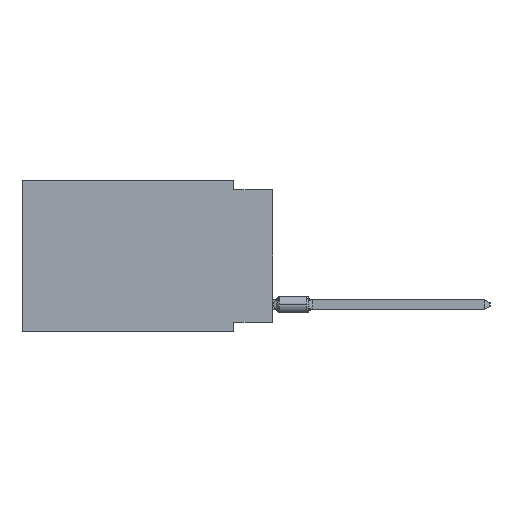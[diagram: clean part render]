
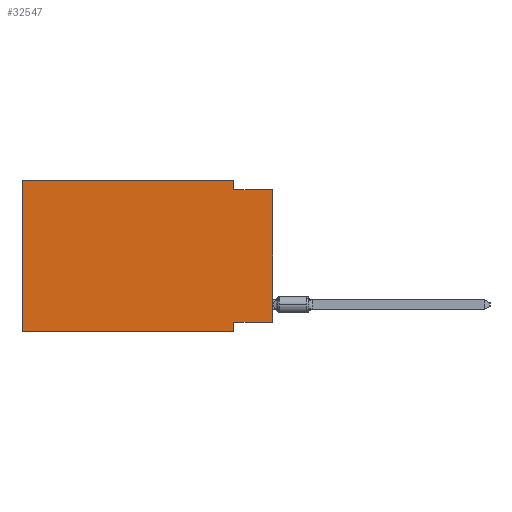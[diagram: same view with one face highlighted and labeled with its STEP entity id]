
A CAD part, left-side view. The second image highlights one B-rep face of the part: STEP entity #32547.
In plain terms, the highlighted planar face has unit normal (-1, 0, 0).
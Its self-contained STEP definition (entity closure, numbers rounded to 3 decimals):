
#384 = VERTEX_POINT ( 'NONE', #21539 ) ;
#2235 = EDGE_CURVE ( 'NONE', #37856, #26172, #39599, .T. ) ;
#2510 = CARTESIAN_POINT ( 'NONE',  ( 0., 16.383, -9.906 ) ) ;
#2633 = CARTESIAN_POINT ( 'NONE',  ( 0., 16.383, 0. ) ) ;
#3604 = CARTESIAN_POINT ( 'NONE',  ( 0., 16.383, 0. ) ) ;
#4137 = DIRECTION ( 'NONE',  ( 0., -1., 0. ) ) ;
#4567 = EDGE_CURVE ( 'NONE', #40803, #26172, #17287, .T. ) ;
#4805 = CARTESIAN_POINT ( 'NONE',  ( 0., 0., -9.271 ) ) ;
#4965 = VECTOR ( 'NONE', #42266, 1000. ) ;
#5378 = CARTESIAN_POINT ( 'NONE',  ( 0., 0., 0. ) ) ;
#6723 = DIRECTION ( 'NONE',  ( 1., 0., 0. ) ) ;
#7190 = ORIENTED_EDGE ( 'NONE', *, *, #26033, .F. ) ;
#9880 = AXIS2_PLACEMENT_3D ( 'NONE', #3604, #6723, #38810 ) ;
#10852 = CARTESIAN_POINT ( 'NONE',  ( 0., 2.54, -9.906 ) ) ;
#11183 = EDGE_LOOP ( 'NONE', ( #23710, #33971, #49296, #17573, #24933, #50683, #7190, #35053 ) ) ;
#11378 = CARTESIAN_POINT ( 'NONE',  ( 0., 2.54, 0. ) ) ;
#11537 = VERTEX_POINT ( 'NONE', #30456 ) ;
#11984 = VERTEX_POINT ( 'NONE', #35717 ) ;
#15639 = EDGE_CURVE ( 'NONE', #11984, #11537, #33184, .T. ) ;
#15803 = CARTESIAN_POINT ( 'NONE',  ( 0., 0., -0.635 ) ) ;
#17287 = LINE ( 'NONE', #5378, #30289 ) ;
#17573 = ORIENTED_EDGE ( 'NONE', *, *, #15639, .F. ) ;
#17664 = DIRECTION ( 'NONE',  ( 0., -1., 0. ) ) ;
#19422 = EDGE_CURVE ( 'NONE', #40803, #384, #34007, .T. ) ;
#21539 = CARTESIAN_POINT ( 'NONE',  ( 0., 2.54, -9.271 ) ) ;
#21634 = CARTESIAN_POINT ( 'NONE',  ( 0., 2.54, -0.635 ) ) ;
#23710 = ORIENTED_EDGE ( 'NONE', *, *, #4567, .T. ) ;
#24933 = ORIENTED_EDGE ( 'NONE', *, *, #29945, .F. ) ;
#26033 = EDGE_CURVE ( 'NONE', #384, #34349, #45617, .T. ) ;
#26172 = VERTEX_POINT ( 'NONE', #44912 ) ;
#26659 = PLANE ( 'NONE',  #9880 ) ;
#26674 = LINE ( 'NONE', #34695, #36196 ) ;
#27167 = VECTOR ( 'NONE', #34433, 1000. ) ;
#29945 = EDGE_CURVE ( 'NONE', #48375, #11984, #26674, .T. ) ;
#30033 = EDGE_CURVE ( 'NONE', #11537, #37856, #31319, .T. ) ;
#30289 = VECTOR ( 'NONE', #36696, 1000. ) ;
#30456 = CARTESIAN_POINT ( 'NONE',  ( 0., 2.54, 0. ) ) ;
#31319 = LINE ( 'NONE', #11378, #27167 ) ;
#31550 = VECTOR ( 'NONE', #17664, 1000. ) ;
#32547 = ADVANCED_FACE ( 'NONE', ( #41922 ), #26659, .F. ) ;
#33184 = LINE ( 'NONE', #2633, #31550 ) ;
#33971 = ORIENTED_EDGE ( 'NONE', *, *, #2235, .F. ) ;
#34007 = LINE ( 'NONE', #49742, #4965 ) ;
#34349 = VERTEX_POINT ( 'NONE', #10852 ) ;
#34433 = DIRECTION ( 'NONE',  ( 0., 0., -1. ) ) ;
#34620 = EDGE_CURVE ( 'NONE', #48375, #34349, #45722, .T. ) ;
#34695 = CARTESIAN_POINT ( 'NONE',  ( 0., 16.383, 0. ) ) ;
#35053 = ORIENTED_EDGE ( 'NONE', *, *, #19422, .F. ) ;
#35717 = CARTESIAN_POINT ( 'NONE',  ( 0., 16.383, 0. ) ) ;
#36196 = VECTOR ( 'NONE', #42928, 1000. ) ;
#36696 = DIRECTION ( 'NONE',  ( 0., 0., 1. ) ) ;
#37856 = VERTEX_POINT ( 'NONE', #21634 ) ;
#38779 = CARTESIAN_POINT ( 'NONE',  ( 0., 16.383, -9.906 ) ) ;
#38810 = DIRECTION ( 'NONE',  ( 0., 0., -1. ) ) ;
#39344 = VECTOR ( 'NONE', #50249, 1000. ) ;
#39599 = LINE ( 'NONE', #15803, #40704 ) ;
#40704 = VECTOR ( 'NONE', #4137, 1000. ) ;
#40803 = VERTEX_POINT ( 'NONE', #4805 ) ;
#41922 = FACE_OUTER_BOUND ( 'NONE', #11183, .T. ) ;
#42266 = DIRECTION ( 'NONE',  ( 0., 1., 0. ) ) ;
#42928 = DIRECTION ( 'NONE',  ( 0., 0., 1. ) ) ;
#43949 = VECTOR ( 'NONE', #49844, 1000. ) ;
#44912 = CARTESIAN_POINT ( 'NONE',  ( 0., 0., -0.635 ) ) ;
#45617 = LINE ( 'NONE', #50501, #39344 ) ;
#45722 = LINE ( 'NONE', #2510, #43949 ) ;
#48375 = VERTEX_POINT ( 'NONE', #38779 ) ;
#49296 = ORIENTED_EDGE ( 'NONE', *, *, #30033, .F. ) ;
#49742 = CARTESIAN_POINT ( 'NONE',  ( 0., 0., -9.271 ) ) ;
#49844 = DIRECTION ( 'NONE',  ( 0., -1., 0. ) ) ;
#50249 = DIRECTION ( 'NONE',  ( 0., 0., -1. ) ) ;
#50501 = CARTESIAN_POINT ( 'NONE',  ( 0., 2.54, -9.906 ) ) ;
#50683 = ORIENTED_EDGE ( 'NONE', *, *, #34620, .T. ) ;
